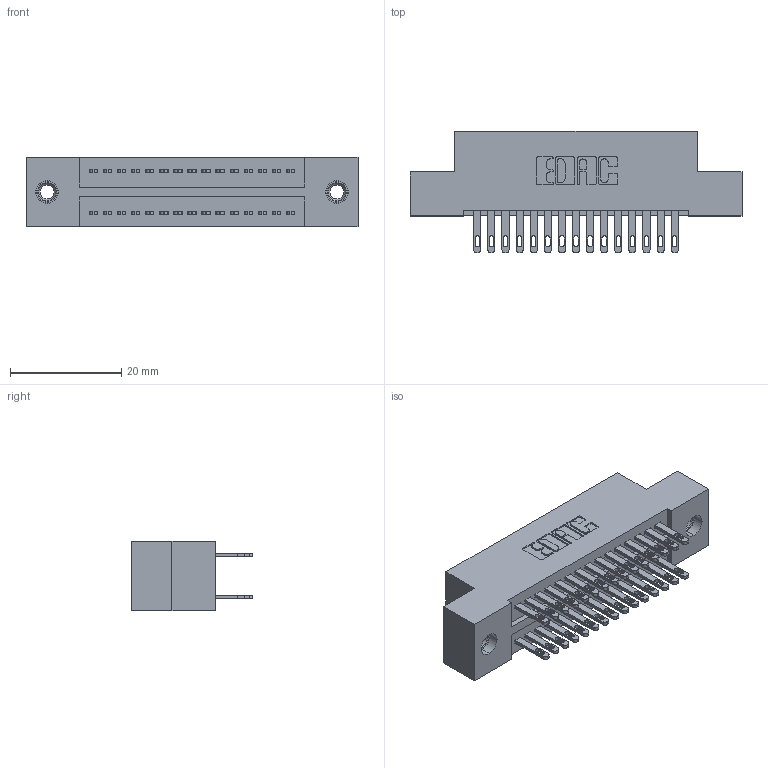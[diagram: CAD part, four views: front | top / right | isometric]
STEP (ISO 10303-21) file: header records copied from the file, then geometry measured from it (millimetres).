
FILE_DESCRIPTION (( 'STEP AP203' ), '1' );
FILE_NAME ('325-030-500-207.STEP', '2020-02-24T19:03:46', ( '' ), ( '' ), 'SwSTEP 2.0', 'SolidWorks 2016', '' );
FILE_SCHEMA (( 'CONFIG_CONTROL_DESIGN' ));
Length unit declared in the file: inch
Products named in the file (4): 345-250-001_345-250-005-103; 325-292-001_325-293-100; 325-030-500-207; 325 Part_TI
Assembly tree (33 placements, depth 2):
  325-030-500-207
    325 Part_TI
    325-292-001_325-293-100  x30
    345-250-001_345-250-005-103  x2
Bounding box: 59.82 x 21.84 x 12.45 mm (x, y, z)
Volume: 7558 mm3; surface area: 8847.6 mm2
Topology: 33 solids, 33 shells, 1614 faces, 4857 edges, 3230 vertices
Faces by surface type: plane 1002, cylinder 596, cone 12, torus 4
Entity records: 14258 total; most frequent: CARTESIAN_POINT 2377, ORIENTED_EDGE 2306, DIRECTION 2111, EDGE_CURVE 1153, LINE 1001, VECTOR 1001, VERTEX_POINT 764, AXIS2_PLACEMENT_3D 555
